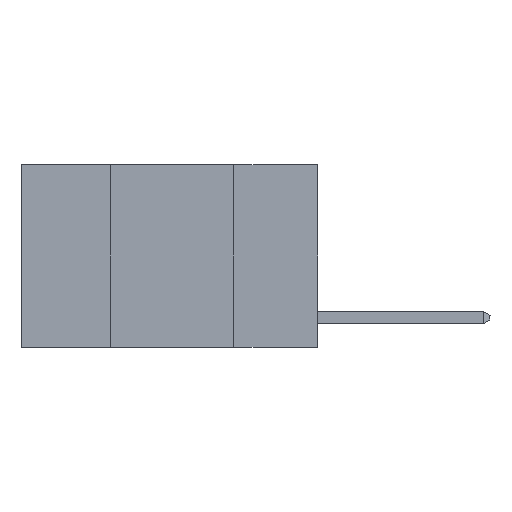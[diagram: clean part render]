
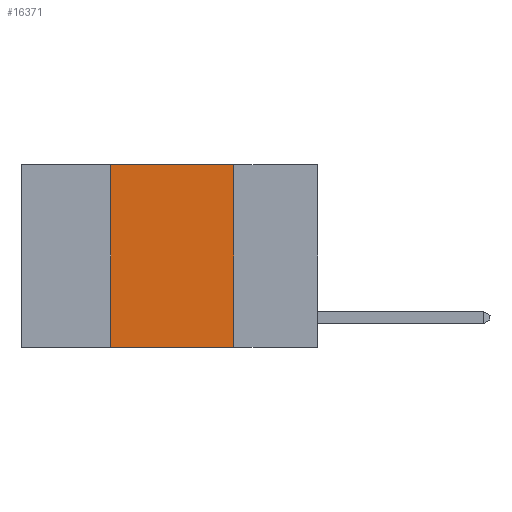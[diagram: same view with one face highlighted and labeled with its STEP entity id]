
A CAD part, left-side view. The second image highlights one B-rep face of the part: STEP entity #16371.
In plain terms, the highlighted planar face has unit normal (-1, 0, 0).
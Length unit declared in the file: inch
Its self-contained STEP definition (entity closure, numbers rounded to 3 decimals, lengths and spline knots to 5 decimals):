
#1252 = ORIENTED_EDGE ( 'NONE', *, *, #4825, .F. ) ;
#1632 = CARTESIAN_POINT ( 'NONE',  ( 0., 0.6, 0. ) ) ;
#1760 = CARTESIAN_POINT ( 'NONE',  ( 0., 0.6, 0. ) ) ;
#2321 = CARTESIAN_POINT ( 'NONE',  ( 0., 0.42, 0. ) ) ;
#3405 = EDGE_CURVE ( 'NONE', #4045, #4860, #20371, .T. ) ;
#3940 = AXIS2_PLACEMENT_3D ( 'NONE', #1760, #6789, #13211 ) ;
#4045 = VERTEX_POINT ( 'NONE', #14724 ) ;
#4352 = EDGE_LOOP ( 'NONE', ( #13554, #1252, #8111, #17863 ) ) ;
#4825 = EDGE_CURVE ( 'NONE', #17439, #16892, #19190, .T. ) ;
#4860 = VERTEX_POINT ( 'NONE', #7171 ) ;
#5384 = VECTOR ( 'NONE', #11189, 39.37008 ) ;
#6477 = CARTESIAN_POINT ( 'NONE',  ( 0., 0.17, 0. ) ) ;
#6597 = PLANE ( 'NONE',  #3940 ) ;
#6789 = DIRECTION ( 'NONE',  ( 1., 0., 0. ) ) ;
#7170 = CARTESIAN_POINT ( 'NONE',  ( 0., 0.17, 0. ) ) ;
#7171 = CARTESIAN_POINT ( 'NONE',  ( 0., 0.17, -0.37 ) ) ;
#7474 = CARTESIAN_POINT ( 'NONE',  ( 0., 0.42, 0. ) ) ;
#7704 = CARTESIAN_POINT ( 'NONE',  ( 0., 0.6, -0.37 ) ) ;
#7909 = DIRECTION ( 'NONE',  ( 0., -1., 0. ) ) ;
#8111 = ORIENTED_EDGE ( 'NONE', *, *, #18402, .F. ) ;
#8715 = EDGE_CURVE ( 'NONE', #16892, #4860, #17924, .T. ) ;
#10741 = VECTOR ( 'NONE', #18024, 39.37008 ) ;
#11189 = DIRECTION ( 'NONE',  ( 0., -1., 0. ) ) ;
#12414 = VECTOR ( 'NONE', #7909, 39.37008 ) ;
#13211 = DIRECTION ( 'NONE',  ( 0., 0., -1. ) ) ;
#13554 = ORIENTED_EDGE ( 'NONE', *, *, #8715, .F. ) ;
#14011 = LINE ( 'NONE', #7474, #17959 ) ;
#14125 = DIRECTION ( 'NONE',  ( 0., 0., 1. ) ) ;
#14724 = CARTESIAN_POINT ( 'NONE',  ( 0., 0.42, -0.37 ) ) ;
#16168 = FACE_OUTER_BOUND ( 'NONE', #4352, .T. ) ;
#16371 = ADVANCED_FACE ( 'NONE', ( #16168 ), #6597, .F. ) ;
#16892 = VERTEX_POINT ( 'NONE', #7170 ) ;
#17439 = VERTEX_POINT ( 'NONE', #2321 ) ;
#17863 = ORIENTED_EDGE ( 'NONE', *, *, #3405, .T. ) ;
#17924 = LINE ( 'NONE', #6477, #10741 ) ;
#17959 = VECTOR ( 'NONE', #14125, 39.37008 ) ;
#18024 = DIRECTION ( 'NONE',  ( 0., 0., -1. ) ) ;
#18402 = EDGE_CURVE ( 'NONE', #4045, #17439, #14011, .T. ) ;
#19190 = LINE ( 'NONE', #1632, #5384 ) ;
#20371 = LINE ( 'NONE', #7704, #12414 ) ;
